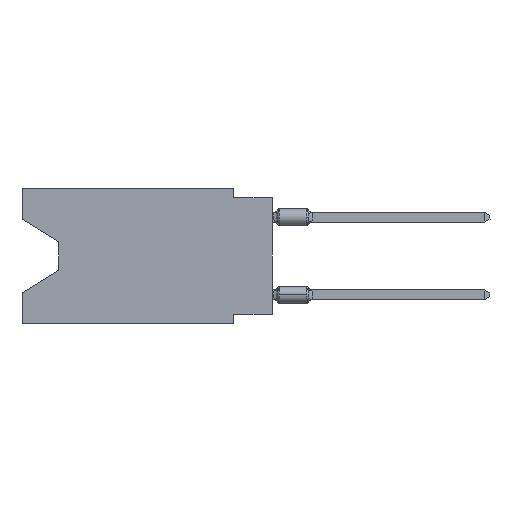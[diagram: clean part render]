
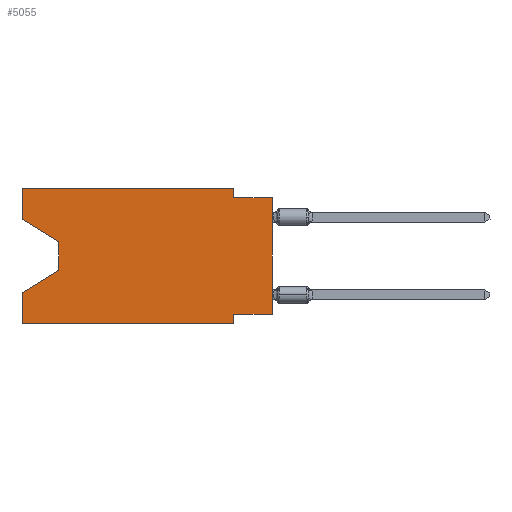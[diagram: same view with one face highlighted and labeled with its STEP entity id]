
A CAD part, left-side view. The second image highlights one B-rep face of the part: STEP entity #5055.
In plain terms, the highlighted planar face has unit normal (-1, 0, 0).
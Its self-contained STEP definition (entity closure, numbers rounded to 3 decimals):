
#20 = DIRECTION ( 'NONE',  ( 0., 0., -1. ) ) ;
#147 = VERTEX_POINT ( 'NONE', #30354 ) ;
#308 = VECTOR ( 'NONE', #25346, 1000. ) ;
#576 = VERTEX_POINT ( 'NONE', #18736 ) ;
#898 = EDGE_CURVE ( 'NONE', #8719, #576, #28367, .T. ) ;
#1033 = LINE ( 'NONE', #3180, #4153 ) ;
#1248 = CARTESIAN_POINT ( 'NONE',  ( 0., 2.54, -8.89 ) ) ;
#1266 = VERTEX_POINT ( 'NONE', #16155 ) ;
#1315 = CARTESIAN_POINT ( 'NONE',  ( 0., 0., -8.255 ) ) ;
#1913 = CARTESIAN_POINT ( 'NONE',  ( 0., 2.54, -8.89 ) ) ;
#1978 = EDGE_CURVE ( 'NONE', #2861, #1266, #3730, .T. ) ;
#2434 = CARTESIAN_POINT ( 'NONE',  ( 0., 16.383, 0. ) ) ;
#2503 = VECTOR ( 'NONE', #19553, 1000. ) ;
#2660 = VECTOR ( 'NONE', #18819, 1000. ) ;
#2861 = VERTEX_POINT ( 'NONE', #1315 ) ;
#3048 = VECTOR ( 'NONE', #24343, 1000. ) ;
#3180 = CARTESIAN_POINT ( 'NONE',  ( 0., 0., 0. ) ) ;
#3475 = CARTESIAN_POINT ( 'NONE',  ( 0., 16.383, 0. ) ) ;
#3567 = CARTESIAN_POINT ( 'NONE',  ( 0., 2.54, 0. ) ) ;
#3643 = DIRECTION ( 'NONE',  ( 0., 0., 1. ) ) ;
#3730 = LINE ( 'NONE', #27506, #22437 ) ;
#4047 = ORIENTED_EDGE ( 'NONE', *, *, #8121, .F. ) ;
#4153 = VECTOR ( 'NONE', #29128, 1000. ) ;
#4535 = ORIENTED_EDGE ( 'NONE', *, *, #898, .T. ) ;
#4744 = DIRECTION ( 'NONE',  ( 0., 0., -1. ) ) ;
#5043 = LINE ( 'NONE', #17573, #3048 ) ;
#5055 = ADVANCED_FACE ( 'NONE', ( #5601 ), #7933, .F. ) ;
#5367 = VECTOR ( 'NONE', #20, 1000. ) ;
#5601 = FACE_OUTER_BOUND ( 'NONE', #22812, .T. ) ;
#7204 = CARTESIAN_POINT ( 'NONE',  ( 0., 16.383, -2.038 ) ) ;
#7455 = VERTEX_POINT ( 'NONE', #22309 ) ;
#7493 = CARTESIAN_POINT ( 'NONE',  ( 0., 0., -0.635 ) ) ;
#7573 = CARTESIAN_POINT ( 'NONE',  ( 0., 13.97, -5.385 ) ) ;
#7806 = LINE ( 'NONE', #2434, #11491 ) ;
#7844 = EDGE_CURVE ( 'NONE', #7455, #147, #29838, .T. ) ;
#7933 = PLANE ( 'NONE',  #23073 ) ;
#8121 = EDGE_CURVE ( 'NONE', #1266, #16172, #19451, .T. ) ;
#8153 = VECTOR ( 'NONE', #21689, 1000. ) ;
#8538 = DIRECTION ( 'NONE',  ( 1., 0., 0. ) ) ;
#8719 = VERTEX_POINT ( 'NONE', #9203 ) ;
#8872 = EDGE_CURVE ( 'NONE', #16211, #147, #12117, .T. ) ;
#9203 = CARTESIAN_POINT ( 'NONE',  ( 0., 16.383, -2.038 ) ) ;
#9607 = VECTOR ( 'NONE', #28879, 1000. ) ;
#10118 = ORIENTED_EDGE ( 'NONE', *, *, #7844, .F. ) ;
#10856 = VECTOR ( 'NONE', #28217, 1000. ) ;
#11491 = VECTOR ( 'NONE', #3643, 1000. ) ;
#12117 = LINE ( 'NONE', #24008, #8153 ) ;
#12223 = ORIENTED_EDGE ( 'NONE', *, *, #24012, .T. ) ;
#12231 = VERTEX_POINT ( 'NONE', #29748 ) ;
#12745 = ORIENTED_EDGE ( 'NONE', *, *, #25219, .F. ) ;
#12889 = EDGE_CURVE ( 'NONE', #576, #16211, #16536, .T. ) ;
#13884 = VERTEX_POINT ( 'NONE', #3475 ) ;
#14795 = ORIENTED_EDGE ( 'NONE', *, *, #17139, .F. ) ;
#15189 = CARTESIAN_POINT ( 'NONE',  ( 0., 16.383, 0. ) ) ;
#15880 = EDGE_CURVE ( 'NONE', #12231, #23529, #17970, .T. ) ;
#16155 = CARTESIAN_POINT ( 'NONE',  ( 0., 2.54, -8.255 ) ) ;
#16172 = VERTEX_POINT ( 'NONE', #1913 ) ;
#16211 = VERTEX_POINT ( 'NONE', #7573 ) ;
#16493 = LINE ( 'NONE', #25904, #27742 ) ;
#16536 = LINE ( 'NONE', #25949, #5367 ) ;
#17139 = EDGE_CURVE ( 'NONE', #19033, #12231, #16493, .T. ) ;
#17573 = CARTESIAN_POINT ( 'NONE',  ( 0., 16.383, -8.89 ) ) ;
#17953 = CARTESIAN_POINT ( 'NONE',  ( 0., 16.383, 0. ) ) ;
#17970 = LINE ( 'NONE', #7493, #2503 ) ;
#18287 = EDGE_CURVE ( 'NONE', #13884, #19033, #23431, .T. ) ;
#18736 = CARTESIAN_POINT ( 'NONE',  ( 0., 13.97, -3.505 ) ) ;
#18819 = DIRECTION ( 'NONE',  ( 0., -1., 0. ) ) ;
#19033 = VERTEX_POINT ( 'NONE', #3567 ) ;
#19451 = LINE ( 'NONE', #1248, #9607 ) ;
#19553 = DIRECTION ( 'NONE',  ( 0., -1., 0. ) ) ;
#19823 = DIRECTION ( 'NONE',  ( 0., 0., -1. ) ) ;
#20454 = ORIENTED_EDGE ( 'NONE', *, *, #8872, .T. ) ;
#20902 = ORIENTED_EDGE ( 'NONE', *, *, #18287, .F. ) ;
#21411 = CARTESIAN_POINT ( 'NONE',  ( 0., 16.383, 0. ) ) ;
#21689 = DIRECTION ( 'NONE',  ( 0., 0.855, -0.519 ) ) ;
#21736 = EDGE_CURVE ( 'NONE', #7455, #16172, #5043, .T. ) ;
#22309 = CARTESIAN_POINT ( 'NONE',  ( 0., 16.383, -8.89 ) ) ;
#22437 = VECTOR ( 'NONE', #29528, 1000. ) ;
#22812 = EDGE_LOOP ( 'NONE', ( #4535, #25383, #20454, #10118, #24621, #4047, #24933, #12223, #23243, #14795, #20902, #12745 ) ) ;
#23073 = AXIS2_PLACEMENT_3D ( 'NONE', #15189, #8538, #19823 ) ;
#23243 = ORIENTED_EDGE ( 'NONE', *, *, #15880, .F. ) ;
#23431 = LINE ( 'NONE', #21411, #2660 ) ;
#23529 = VERTEX_POINT ( 'NONE', #26834 ) ;
#24008 = CARTESIAN_POINT ( 'NONE',  ( 0., 13.97, -5.385 ) ) ;
#24012 = EDGE_CURVE ( 'NONE', #2861, #23529, #1033, .T. ) ;
#24343 = DIRECTION ( 'NONE',  ( 0., -1., 0. ) ) ;
#24621 = ORIENTED_EDGE ( 'NONE', *, *, #21736, .T. ) ;
#24933 = ORIENTED_EDGE ( 'NONE', *, *, #1978, .F. ) ;
#25219 = EDGE_CURVE ( 'NONE', #8719, #13884, #7806, .T. ) ;
#25346 = DIRECTION ( 'NONE',  ( 0., 0., 1. ) ) ;
#25383 = ORIENTED_EDGE ( 'NONE', *, *, #12889, .T. ) ;
#25904 = CARTESIAN_POINT ( 'NONE',  ( 0., 2.54, 0. ) ) ;
#25949 = CARTESIAN_POINT ( 'NONE',  ( 0., 13.97, -3.505 ) ) ;
#26834 = CARTESIAN_POINT ( 'NONE',  ( 0., 0., -0.635 ) ) ;
#27506 = CARTESIAN_POINT ( 'NONE',  ( 0., 0., -8.255 ) ) ;
#27742 = VECTOR ( 'NONE', #4744, 1000. ) ;
#28217 = DIRECTION ( 'NONE',  ( 0., -0.855, -0.519 ) ) ;
#28367 = LINE ( 'NONE', #7204, #10856 ) ;
#28879 = DIRECTION ( 'NONE',  ( 0., 0., -1. ) ) ;
#29128 = DIRECTION ( 'NONE',  ( 0., 0., 1. ) ) ;
#29528 = DIRECTION ( 'NONE',  ( 0., 1., 0. ) ) ;
#29748 = CARTESIAN_POINT ( 'NONE',  ( 0., 2.54, -0.635 ) ) ;
#29838 = LINE ( 'NONE', #17953, #308 ) ;
#30354 = CARTESIAN_POINT ( 'NONE',  ( 0., 16.383, -6.852 ) ) ;
